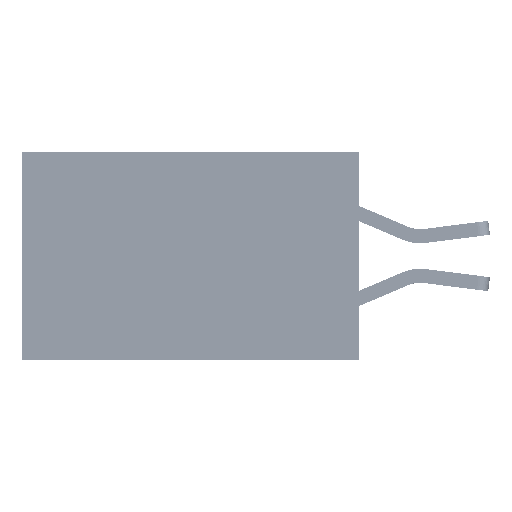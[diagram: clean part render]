
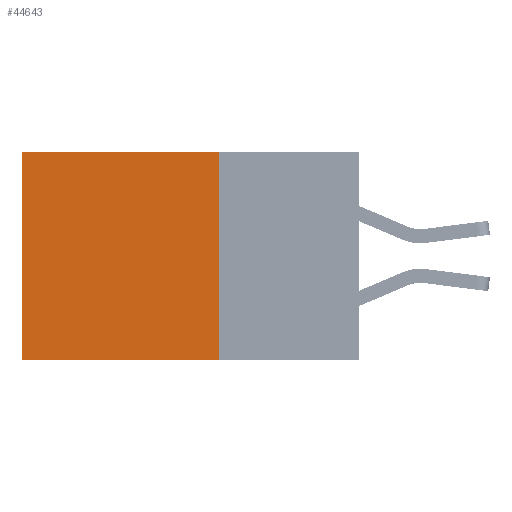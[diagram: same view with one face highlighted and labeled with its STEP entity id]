
A CAD part, left-side view. The second image highlights one B-rep face of the part: STEP entity #44643.
In plain terms, the highlighted planar face has unit normal (-1, 0, 0).
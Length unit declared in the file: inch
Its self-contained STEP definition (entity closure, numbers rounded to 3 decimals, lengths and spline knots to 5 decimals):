
#1160 = CARTESIAN_POINT ( 'NONE',  ( 0.2875, 0.25, 0. ) ) ;
#1445 = VERTEX_POINT ( 'NONE', #42376 ) ;
#2978 = CARTESIAN_POINT ( 'NONE',  ( 0.2875, 0.25, -0.37 ) ) ;
#4076 = EDGE_CURVE ( 'NONE', #17152, #1445, #30121, .T. ) ;
#4720 = DIRECTION ( 'NONE',  ( 0., 0., -1. ) ) ;
#5251 = EDGE_CURVE ( 'NONE', #16607, #17152, #39670, .T. ) ;
#5387 = LINE ( 'NONE', #30509, #21942 ) ;
#5948 = CARTESIAN_POINT ( 'NONE',  ( 0.2875, 0.25, 0. ) ) ;
#7740 = VECTOR ( 'NONE', #12911, 39.37008 ) ;
#9453 = DIRECTION ( 'NONE',  ( 0., 0., -1. ) ) ;
#11685 = VECTOR ( 'NONE', #44330, 39.37008 ) ;
#12911 = DIRECTION ( 'NONE',  ( 0., 1., 0. ) ) ;
#13576 = EDGE_LOOP ( 'NONE', ( #43665, #15785, #36782, #39049 ) ) ;
#15785 = ORIENTED_EDGE ( 'NONE', *, *, #4076, .F. ) ;
#16607 = VERTEX_POINT ( 'NONE', #5948 ) ;
#17152 = VERTEX_POINT ( 'NONE', #19199 ) ;
#18297 = VERTEX_POINT ( 'NONE', #29496 ) ;
#19199 = CARTESIAN_POINT ( 'NONE',  ( 0.2875, 0.25, -0.37 ) ) ;
#20811 = VECTOR ( 'NONE', #31177, 39.37008 ) ;
#21916 = EDGE_CURVE ( 'NONE', #16607, #18297, #24272, .T. ) ;
#21942 = VECTOR ( 'NONE', #9453, 39.37008 ) ;
#23607 = AXIS2_PLACEMENT_3D ( 'NONE', #1160, #25805, #4720 ) ;
#24272 = LINE ( 'NONE', #33892, #7740 ) ;
#25721 = EDGE_CURVE ( 'NONE', #18297, #1445, #5387, .T. ) ;
#25805 = DIRECTION ( 'NONE',  ( 1., 0., 0. ) ) ;
#29496 = CARTESIAN_POINT ( 'NONE',  ( 0.2875, 0.6, 0. ) ) ;
#30121 = LINE ( 'NONE', #2978, #20811 ) ;
#30509 = CARTESIAN_POINT ( 'NONE',  ( 0.2875, 0.6, 0. ) ) ;
#31177 = DIRECTION ( 'NONE',  ( 0., 1., 0. ) ) ;
#33682 = CARTESIAN_POINT ( 'NONE',  ( 0.2875, 0.25, 0. ) ) ;
#33892 = CARTESIAN_POINT ( 'NONE',  ( 0.2875, 0.25, 0. ) ) ;
#34570 = FACE_OUTER_BOUND ( 'NONE', #13576, .T. ) ;
#36257 = PLANE ( 'NONE',  #23607 ) ;
#36782 = ORIENTED_EDGE ( 'NONE', *, *, #5251, .F. ) ;
#39049 = ORIENTED_EDGE ( 'NONE', *, *, #21916, .T. ) ;
#39670 = LINE ( 'NONE', #33682, #11685 ) ;
#42376 = CARTESIAN_POINT ( 'NONE',  ( 0.2875, 0.6, -0.37 ) ) ;
#43665 = ORIENTED_EDGE ( 'NONE', *, *, #25721, .T. ) ;
#44330 = DIRECTION ( 'NONE',  ( 0., 0., -1. ) ) ;
#44643 = ADVANCED_FACE ( 'NONE', ( #34570 ), #36257, .F. ) ;
